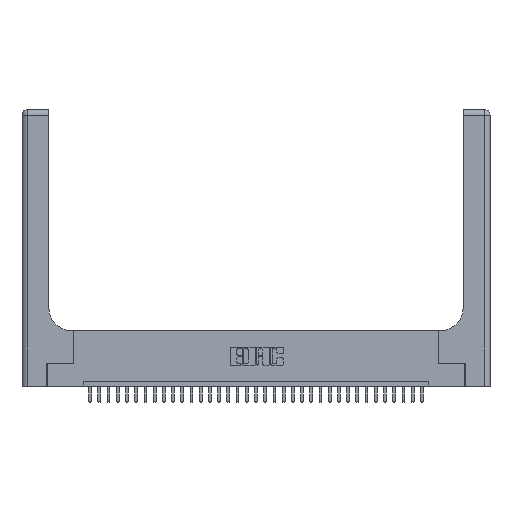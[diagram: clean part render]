
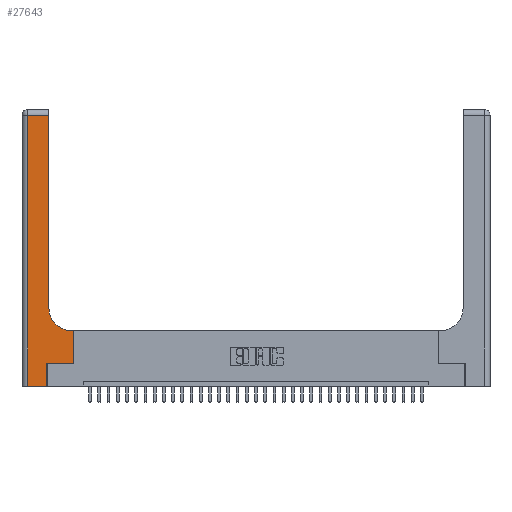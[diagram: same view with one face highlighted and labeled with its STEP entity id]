
A CAD part, top view. The second image highlights one B-rep face of the part: STEP entity #27643.
In plain terms, the highlighted planar face has unit normal (0, 0, 1).
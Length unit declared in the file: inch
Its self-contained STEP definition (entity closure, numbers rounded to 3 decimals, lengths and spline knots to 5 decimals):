
#631 = VERTEX_POINT ( 'NONE', #25679 ) ;
#1587 = LINE ( 'NONE', #3513, #7664 ) ;
#2075 = VECTOR ( 'NONE', #16801, 39.37008 ) ;
#2357 = VERTEX_POINT ( 'NONE', #32848 ) ;
#2719 = VERTEX_POINT ( 'NONE', #30174 ) ;
#2851 = EDGE_CURVE ( 'NONE', #29460, #6004, #7046, .T. ) ;
#2936 = DIRECTION ( 'NONE',  ( 0., 1., 0. ) ) ;
#3513 = CARTESIAN_POINT ( 'NONE',  ( 0.269, 0.25, 0.37 ) ) ;
#4326 = DIRECTION ( 'NONE',  ( 1., 0., 0. ) ) ;
#4733 = EDGE_CURVE ( 'NONE', #11427, #5722, #32705, .T. ) ;
#5669 = VERTEX_POINT ( 'NONE', #32303 ) ;
#5685 = EDGE_CURVE ( 'NONE', #23271, #2357, #1587, .T. ) ;
#5722 = VERTEX_POINT ( 'NONE', #25178 ) ;
#5764 = EDGE_CURVE ( 'NONE', #5722, #5669, #28523, .T. ) ;
#5902 = EDGE_CURVE ( 'NONE', #6004, #631, #24810, .T. ) ;
#6004 = VERTEX_POINT ( 'NONE', #15708 ) ;
#6096 = VECTOR ( 'NONE', #26014, 39.37008 ) ;
#6828 = EDGE_CURVE ( 'NONE', #631, #11427, #21881, .T. ) ;
#7046 = CIRCLE ( 'NONE', #17150, 0.25 ) ;
#7175 = CARTESIAN_POINT ( 'NONE',  ( 0.5415, 0.6, 0.37 ) ) ;
#7543 = EDGE_CURVE ( 'NONE', #2357, #2719, #30049, .T. ) ;
#7664 = VECTOR ( 'NONE', #26907, 39.37008 ) ;
#7985 = VECTOR ( 'NONE', #16790, 39.37008 ) ;
#8848 = AXIS2_PLACEMENT_3D ( 'NONE', #25894, #28089, #28333 ) ;
#8897 = LINE ( 'NONE', #33808, #6096 ) ;
#9089 = CARTESIAN_POINT ( 'NONE',  ( 0.5415, 0.85, 0.37 ) ) ;
#10153 = VECTOR ( 'NONE', #2936, 39.37008 ) ;
#10169 = PLANE ( 'NONE',  #8848 ) ;
#11427 = VERTEX_POINT ( 'NONE', #22065 ) ;
#12389 = ORIENTED_EDGE ( 'NONE', *, *, #4733, .T. ) ;
#12978 = VECTOR ( 'NONE', #4326, 39.37008 ) ;
#15177 = EDGE_CURVE ( 'NONE', #5669, #23271, #33025, .T. ) ;
#15708 = CARTESIAN_POINT ( 'NONE',  ( 0.2915, 0.85, 0.37 ) ) ;
#16174 = CARTESIAN_POINT ( 'NONE',  ( 0.269, 0., 0.37 ) ) ;
#16790 = DIRECTION ( 'NONE',  ( -1., 0., 0. ) ) ;
#16801 = DIRECTION ( 'NONE',  ( 0., -1., 0. ) ) ;
#16956 = DIRECTION ( 'NONE',  ( 1., 0., 0. ) ) ;
#16997 = CARTESIAN_POINT ( 'NONE',  ( 0., 2.94, 0.37 ) ) ;
#17150 = AXIS2_PLACEMENT_3D ( 'NONE', #9089, #27220, #16956 ) ;
#17636 = FACE_OUTER_BOUND ( 'NONE', #31980, .T. ) ;
#18031 = ORIENTED_EDGE ( 'NONE', *, *, #7543, .T. ) ;
#21002 = VECTOR ( 'NONE', #24450, 39.37008 ) ;
#21881 = LINE ( 'NONE', #16997, #7985 ) ;
#21941 = CARTESIAN_POINT ( 'NONE',  ( 0.269, 0.25, 0.37 ) ) ;
#21970 = EDGE_CURVE ( 'NONE', #2719, #29460, #8897, .T. ) ;
#22065 = CARTESIAN_POINT ( 'NONE',  ( 0.06, 2.94, 0.37 ) ) ;
#22419 = ORIENTED_EDGE ( 'NONE', *, *, #21970, .T. ) ;
#23271 = VERTEX_POINT ( 'NONE', #21941 ) ;
#23370 = ORIENTED_EDGE ( 'NONE', *, *, #5902, .T. ) ;
#23530 = ORIENTED_EDGE ( 'NONE', *, *, #6828, .T. ) ;
#23963 = VECTOR ( 'NONE', #30691, 39.37008 ) ;
#24333 = CARTESIAN_POINT ( 'NONE',  ( 0.5585, 0.25, 0.37 ) ) ;
#24450 = DIRECTION ( 'NONE',  ( 0., 1., 0. ) ) ;
#24810 = LINE ( 'NONE', #30577, #23963 ) ;
#25178 = CARTESIAN_POINT ( 'NONE',  ( 0.06, 0., 0.37 ) ) ;
#25679 = CARTESIAN_POINT ( 'NONE',  ( 0.2915, 2.94, 0.37 ) ) ;
#25806 = ORIENTED_EDGE ( 'NONE', *, *, #5685, .T. ) ;
#25894 = CARTESIAN_POINT ( 'NONE',  ( 0., 3., 0.37 ) ) ;
#26014 = DIRECTION ( 'NONE',  ( -1., 0., 0. ) ) ;
#26907 = DIRECTION ( 'NONE',  ( 1., 0., 0. ) ) ;
#27220 = DIRECTION ( 'NONE',  ( 0., 0., -1. ) ) ;
#27643 = ADVANCED_FACE ( 'NONE', ( #17636 ), #10169, .F. ) ;
#27822 = ORIENTED_EDGE ( 'NONE', *, *, #15177, .T. ) ;
#28089 = DIRECTION ( 'NONE',  ( 0., 0., -1. ) ) ;
#28333 = DIRECTION ( 'NONE',  ( -1., 0., 0. ) ) ;
#28523 = LINE ( 'NONE', #32417, #12978 ) ;
#29460 = VERTEX_POINT ( 'NONE', #7175 ) ;
#29485 = ORIENTED_EDGE ( 'NONE', *, *, #5764, .T. ) ;
#29585 = CARTESIAN_POINT ( 'NONE',  ( 0.06, 3., 0.37 ) ) ;
#30049 = LINE ( 'NONE', #24333, #21002 ) ;
#30174 = CARTESIAN_POINT ( 'NONE',  ( 0.5585, 0.6, 0.37 ) ) ;
#30577 = CARTESIAN_POINT ( 'NONE',  ( 0.2915, 3., 0.37 ) ) ;
#30691 = DIRECTION ( 'NONE',  ( 0., 1., 0. ) ) ;
#31980 = EDGE_LOOP ( 'NONE', ( #23370, #23530, #12389, #29485, #27822, #25806, #18031, #22419, #33513 ) ) ;
#32303 = CARTESIAN_POINT ( 'NONE',  ( 0.269, 0., 0.37 ) ) ;
#32417 = CARTESIAN_POINT ( 'NONE',  ( 0., 0., 0.37 ) ) ;
#32705 = LINE ( 'NONE', #29585, #2075 ) ;
#32848 = CARTESIAN_POINT ( 'NONE',  ( 0.5585, 0.25, 0.37 ) ) ;
#33025 = LINE ( 'NONE', #16174, #10153 ) ;
#33513 = ORIENTED_EDGE ( 'NONE', *, *, #2851, .T. ) ;
#33808 = CARTESIAN_POINT ( 'NONE',  ( 0.2915, 0.6, 0.37 ) ) ;
